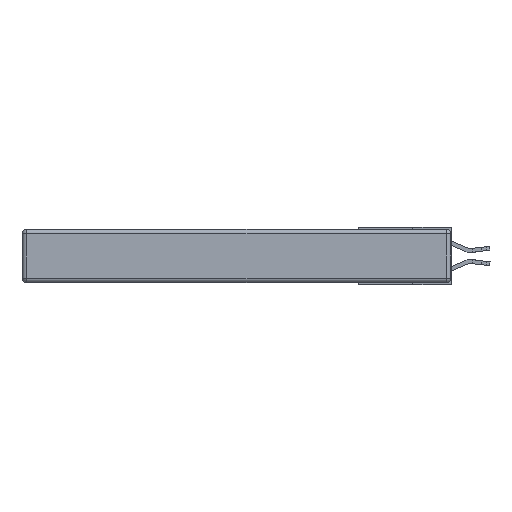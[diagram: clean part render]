
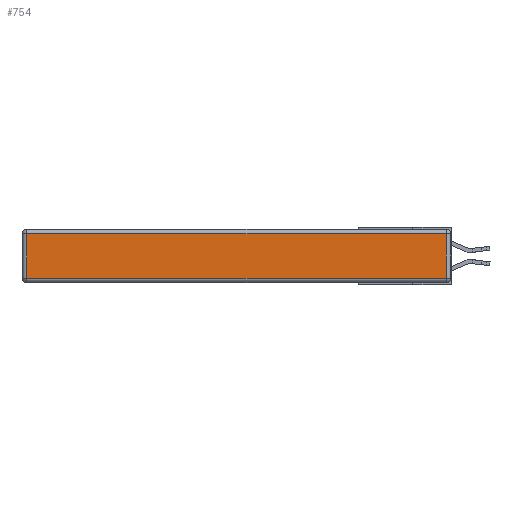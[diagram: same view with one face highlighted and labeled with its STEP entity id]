
A CAD part, left-side view. The second image highlights one B-rep face of the part: STEP entity #754.
In plain terms, the highlighted planar face has unit normal (-1, 0, 0).
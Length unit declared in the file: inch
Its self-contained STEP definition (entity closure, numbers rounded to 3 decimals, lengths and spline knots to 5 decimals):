
#754 = ADVANCED_FACE ( 'NONE', ( #9010 ), #15567, .T. ) ;
#3750 = CARTESIAN_POINT ( 'NONE',  ( 0., 0.03, -0.03 ) ) ;
#4068 = CARTESIAN_POINT ( 'NONE',  ( 0., 0.03, -0.313 ) ) ;
#4224 = CARTESIAN_POINT ( 'NONE',  ( 0., 2.72, -0.03 ) ) ;
#4976 = EDGE_CURVE ( 'NONE', #7976, #15091, #10495, .T. ) ;
#5022 = VERTEX_POINT ( 'NONE', #3750 ) ;
#5889 = CARTESIAN_POINT ( 'NONE',  ( 0., 2.72, -0.313 ) ) ;
#6244 = EDGE_CURVE ( 'NONE', #5022, #12374, #7375, .T. ) ;
#6430 = DIRECTION ( 'NONE',  ( 0., 0., 1. ) ) ;
#6633 = DIRECTION ( 'NONE',  ( 0., -1., 0. ) ) ;
#6690 = DIRECTION ( 'NONE',  ( -1., 0., 0. ) ) ;
#7375 = LINE ( 'NONE', #15578, #8560 ) ;
#7535 = EDGE_CURVE ( 'NONE', #12374, #7976, #9454, .T. ) ;
#7976 = VERTEX_POINT ( 'NONE', #5889 ) ;
#8085 = DIRECTION ( 'NONE',  ( 0., 1., 0. ) ) ;
#8560 = VECTOR ( 'NONE', #8085, 39.37008 ) ;
#9010 = FACE_OUTER_BOUND ( 'NONE', #9118, .T. ) ;
#9118 = EDGE_LOOP ( 'NONE', ( #13565, #16058, #18750, #16092 ) ) ;
#9454 = LINE ( 'NONE', #11085, #18132 ) ;
#10092 = LINE ( 'NONE', #15443, #11736 ) ;
#10495 = LINE ( 'NONE', #15635, #19422 ) ;
#11085 = CARTESIAN_POINT ( 'NONE',  ( 0., 2.72, -0.343 ) ) ;
#11736 = VECTOR ( 'NONE', #6430, 39.37008 ) ;
#12374 = VERTEX_POINT ( 'NONE', #4224 ) ;
#12861 = DIRECTION ( 'NONE',  ( 0., 0., 1. ) ) ;
#13565 = ORIENTED_EDGE ( 'NONE', *, *, #4976, .T. ) ;
#14124 = DIRECTION ( 'NONE',  ( 0., 0., -1. ) ) ;
#14321 = CARTESIAN_POINT ( 'NONE',  ( 0., 0., -0.343 ) ) ;
#15040 = EDGE_CURVE ( 'NONE', #15091, #5022, #10092, .T. ) ;
#15091 = VERTEX_POINT ( 'NONE', #4068 ) ;
#15443 = CARTESIAN_POINT ( 'NONE',  ( 0., 0.03, -0.343 ) ) ;
#15567 = PLANE ( 'NONE',  #17192 ) ;
#15578 = CARTESIAN_POINT ( 'NONE',  ( 0., 2.75, -0.03 ) ) ;
#15635 = CARTESIAN_POINT ( 'NONE',  ( 0., 0., -0.313 ) ) ;
#16058 = ORIENTED_EDGE ( 'NONE', *, *, #15040, .T. ) ;
#16092 = ORIENTED_EDGE ( 'NONE', *, *, #7535, .T. ) ;
#17192 = AXIS2_PLACEMENT_3D ( 'NONE', #14321, #6690, #12861 ) ;
#18132 = VECTOR ( 'NONE', #14124, 39.37008 ) ;
#18750 = ORIENTED_EDGE ( 'NONE', *, *, #6244, .T. ) ;
#19422 = VECTOR ( 'NONE', #6633, 39.37008 ) ;
